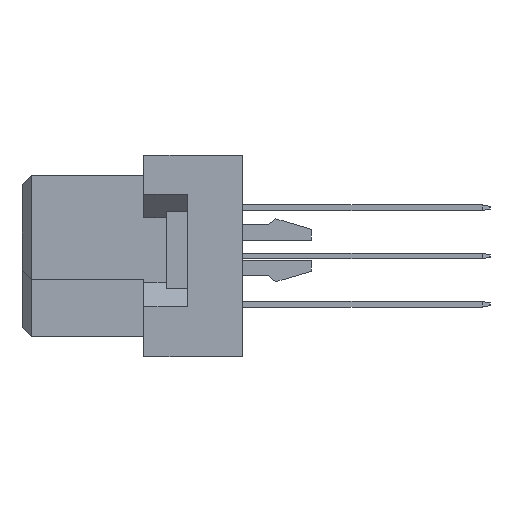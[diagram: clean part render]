
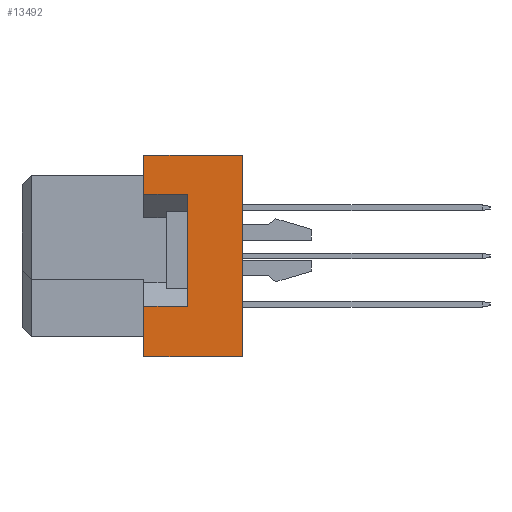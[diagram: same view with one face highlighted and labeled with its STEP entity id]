
A CAD part, left-side view. The second image highlights one B-rep face of the part: STEP entity #13492.
In plain terms, the highlighted planar face has unit normal (-1, 0, 0).
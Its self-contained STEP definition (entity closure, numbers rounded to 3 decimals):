
#549 = VERTEX_POINT ( 'NONE', #24541 ) ;
#644 = CARTESIAN_POINT ( 'NONE',  ( -47.5, -6.4, -2.65 ) ) ;
#745 = ORIENTED_EDGE ( 'NONE', *, *, #13563, .F. ) ;
#929 = VECTOR ( 'NONE', #9023, 1000. ) ;
#1004 = VECTOR ( 'NONE', #18446, 1000. ) ;
#2084 = ORIENTED_EDGE ( 'NONE', *, *, #4703, .F. ) ;
#2482 = LINE ( 'NONE', #24752, #1004 ) ;
#2707 = ORIENTED_EDGE ( 'NONE', *, *, #21233, .T. ) ;
#3131 = DIRECTION ( 'NONE',  ( -1., 0., 0. ) ) ;
#3329 = DIRECTION ( 'NONE',  ( 0., 0., 1. ) ) ;
#3945 = LINE ( 'NONE', #20123, #27893 ) ;
#4281 = CARTESIAN_POINT ( 'NONE',  ( -47.5, -8.7, -2.65 ) ) ;
#4293 = ORIENTED_EDGE ( 'NONE', *, *, #27511, .T. ) ;
#4703 = EDGE_CURVE ( 'NONE', #549, #15311, #2482, .T. ) ;
#5975 = CARTESIAN_POINT ( 'NONE',  ( -47.5, -8.7, -2.65 ) ) ;
#9023 = DIRECTION ( 'NONE',  ( 0., 0., 1. ) ) ;
#11202 = LINE ( 'NONE', #4281, #39998 ) ;
#12225 = VECTOR ( 'NONE', #3329, 1000. ) ;
#12238 = CARTESIAN_POINT ( 'NONE',  ( -47.5, -8.7, -2.65 ) ) ;
#13492 = ADVANCED_FACE ( 'NONE', ( #28754 ), #37635, .T. ) ;
#13563 = EDGE_CURVE ( 'NONE', #20505, #13711, #16990, .T. ) ;
#13711 = VERTEX_POINT ( 'NONE', #24306 ) ;
#15256 = EDGE_CURVE ( 'NONE', #549, #19973, #17856, .T. ) ;
#15311 = VERTEX_POINT ( 'NONE', #34039 ) ;
#16150 = CARTESIAN_POINT ( 'NONE',  ( -47.5, -6.4, -5.3 ) ) ;
#16297 = ORIENTED_EDGE ( 'NONE', *, *, #27202, .F. ) ;
#16787 = ORIENTED_EDGE ( 'NONE', *, *, #15256, .T. ) ;
#16990 = LINE ( 'NONE', #16150, #12225 ) ;
#17140 = VERTEX_POINT ( 'NONE', #5975 ) ;
#17149 = ORIENTED_EDGE ( 'NONE', *, *, #30550, .F. ) ;
#17678 = LINE ( 'NONE', #20443, #25606 ) ;
#17856 = LINE ( 'NONE', #30865, #929 ) ;
#18446 = DIRECTION ( 'NONE',  ( 0., 1., 0. ) ) ;
#18553 = DIRECTION ( 'NONE',  ( 0., 0., 1. ) ) ;
#19973 = VERTEX_POINT ( 'NONE', #39178 ) ;
#20123 = CARTESIAN_POINT ( 'NONE',  ( -47.5, -8.7, 3.25 ) ) ;
#20443 = CARTESIAN_POINT ( 'NONE',  ( -47.5, -6.4, -5.3 ) ) ;
#20468 = DIRECTION ( 'NONE',  ( 0., 1., 0. ) ) ;
#20505 = VERTEX_POINT ( 'NONE', #36386 ) ;
#20556 = CARTESIAN_POINT ( 'NONE',  ( -47.5, -11.6, 5.3 ) ) ;
#20595 = EDGE_LOOP ( 'NONE', ( #2707, #16297, #2084, #16787, #4293, #745, #34668, #17149 ) ) ;
#20643 = VERTEX_POINT ( 'NONE', #28364 ) ;
#21233 = EDGE_CURVE ( 'NONE', #17140, #32526, #11202, .T. ) ;
#21678 = CARTESIAN_POINT ( 'NONE',  ( -47.5, -11.6, 5.3 ) ) ;
#23495 = LINE ( 'NONE', #20556, #41028 ) ;
#23694 = DIRECTION ( 'NONE',  ( 0., 1., 0. ) ) ;
#24306 = CARTESIAN_POINT ( 'NONE',  ( -47.5, -6.4, 5.3 ) ) ;
#24541 = CARTESIAN_POINT ( 'NONE',  ( -47.5, -11.6, -5.3 ) ) ;
#24752 = CARTESIAN_POINT ( 'NONE',  ( -47.5, -11.6, -5.3 ) ) ;
#25606 = VECTOR ( 'NONE', #27541, 1000. ) ;
#25783 = VECTOR ( 'NONE', #18553, 1000. ) ;
#27202 = EDGE_CURVE ( 'NONE', #15311, #32526, #17678, .T. ) ;
#27350 = DIRECTION ( 'NONE',  ( 0., 0., 1. ) ) ;
#27511 = EDGE_CURVE ( 'NONE', #19973, #13711, #23495, .T. ) ;
#27541 = DIRECTION ( 'NONE',  ( 0., 0., 1. ) ) ;
#27617 = AXIS2_PLACEMENT_3D ( 'NONE', #21678, #3131, #27350 ) ;
#27893 = VECTOR ( 'NONE', #37036, 1000. ) ;
#28364 = CARTESIAN_POINT ( 'NONE',  ( -47.5, -8.7, 3.25 ) ) ;
#28754 = FACE_OUTER_BOUND ( 'NONE', #20595, .T. ) ;
#30550 = EDGE_CURVE ( 'NONE', #17140, #20643, #37862, .T. ) ;
#30865 = CARTESIAN_POINT ( 'NONE',  ( -47.5, -11.6, 5.3 ) ) ;
#32526 = VERTEX_POINT ( 'NONE', #644 ) ;
#32922 = EDGE_CURVE ( 'NONE', #20643, #20505, #3945, .T. ) ;
#34039 = CARTESIAN_POINT ( 'NONE',  ( -47.5, -6.4, -5.3 ) ) ;
#34668 = ORIENTED_EDGE ( 'NONE', *, *, #32922, .F. ) ;
#36386 = CARTESIAN_POINT ( 'NONE',  ( -47.5, -6.4, 3.25 ) ) ;
#37036 = DIRECTION ( 'NONE',  ( 0., 1., 0. ) ) ;
#37635 = PLANE ( 'NONE',  #27617 ) ;
#37862 = LINE ( 'NONE', #12238, #25783 ) ;
#39178 = CARTESIAN_POINT ( 'NONE',  ( -47.5, -11.6, 5.3 ) ) ;
#39998 = VECTOR ( 'NONE', #20468, 1000. ) ;
#41028 = VECTOR ( 'NONE', #23694, 1000. ) ;
